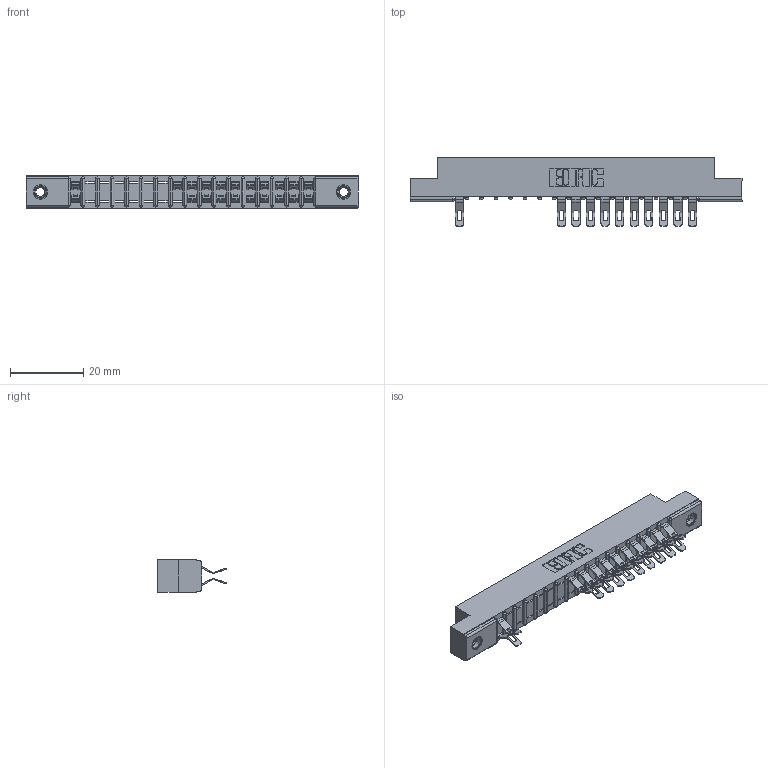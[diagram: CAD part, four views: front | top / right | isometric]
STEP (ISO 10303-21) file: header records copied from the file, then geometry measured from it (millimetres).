
FILE_DESCRIPTION (( 'STEP AP203' ), '1' );
FILE_NAME ('307-034-555-207.STEP', '2018-08-05T06:35:09', ( '' ), ( '' ), 'SwSTEP 2.0', 'SolidWorks 2016', '' );
FILE_SCHEMA (( 'CONFIG_CONTROL_DESIGN' ));
Length unit declared in the file: inch
Products named in the file (4): 307 Part_.156 Dia Mounting Holes; 307-290-001_555; 345-250-001_345-250-005-103; 307-034-555-207
Assembly tree (24 placements, depth 2):
  307-034-555-207
    307 Part_.156 Dia Mounting Holes
    307-290-001_555  x21
    345-250-001_345-250-005-103  x2
Bounding box: 90.37 x 18.75 x 8.71 mm (x, y, z)
Volume: 5792.7 mm3; surface area: 9360.2 mm2
Topology: 24 solids, 24 shells, 1607 faces, 4676 edges, 3032 vertices
Faces by surface type: plane 894, cylinder 661, sphere 36, cone 12, torus 4
Entity records: 19506 total; most frequent: CARTESIAN_POINT 3243, ORIENTED_EDGE 3220, DIRECTION 3190, EDGE_CURVE 1610, VECTOR 1212, LINE 1212, VERTEX_POINT 1042, AXIS2_PLACEMENT_3D 989
